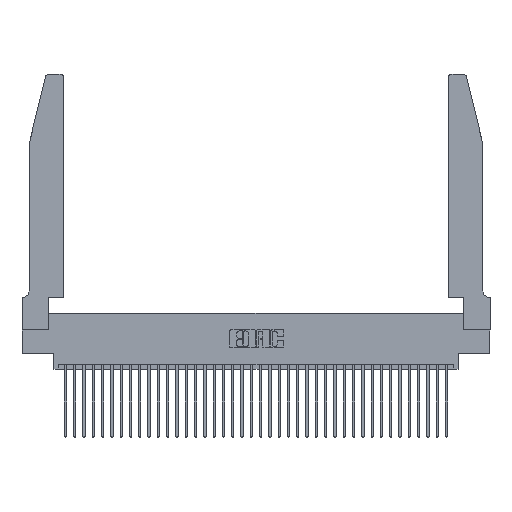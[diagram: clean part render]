
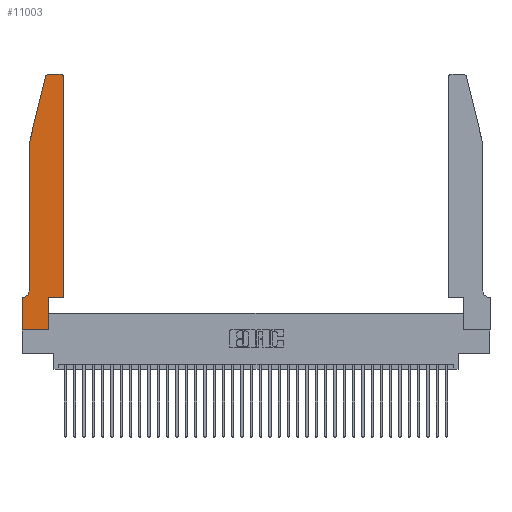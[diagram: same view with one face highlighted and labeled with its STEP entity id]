
A CAD part, top view. The second image highlights one B-rep face of the part: STEP entity #11003.
In plain terms, the highlighted planar face has unit normal (0, 0, 1).
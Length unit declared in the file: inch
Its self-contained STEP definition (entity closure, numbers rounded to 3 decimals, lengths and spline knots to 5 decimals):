
#832 = ORIENTED_EDGE ( 'NONE', *, *, #33440, .T. ) ;
#1424 = EDGE_CURVE ( 'NONE', #3876, #11485, #14101, .T. ) ;
#1878 = VERTEX_POINT ( 'NONE', #6784 ) ;
#2233 = CARTESIAN_POINT ( 'NONE',  ( 0.284, 2.72, 0.37 ) ) ;
#2741 = ORIENTED_EDGE ( 'NONE', *, *, #3928, .T. ) ;
#2839 = AXIS2_PLACEMENT_3D ( 'NONE', #22052, #4454, #24951 ) ;
#3069 = EDGE_CURVE ( 'NONE', #10804, #29101, #21319, .T. ) ;
#3158 = ORIENTED_EDGE ( 'NONE', *, *, #24861, .T. ) ;
#3251 = AXIS2_PLACEMENT_3D ( 'NONE', #17325, #37591, #20279 ) ;
#3876 = VERTEX_POINT ( 'NONE', #34049 ) ;
#3928 = EDGE_CURVE ( 'NONE', #26043, #23030, #18010, .T. ) ;
#4100 = DIRECTION ( 'NONE',  ( 0., 0., 1. ) ) ;
#4180 = CARTESIAN_POINT ( 'NONE',  ( 0.0755, 0.35, 0.37 ) ) ;
#4454 = DIRECTION ( 'NONE',  ( 0., 0., 1. ) ) ;
#5095 = LINE ( 'NONE', #15193, #26618 ) ;
#5207 = DIRECTION ( 'NONE',  ( 1., 0., 0. ) ) ;
#5394 = FACE_OUTER_BOUND ( 'NONE', #14631, .T. ) ;
#5674 = LINE ( 'NONE', #16334, #27212 ) ;
#6263 = VECTOR ( 'NONE', #13726, 39.37008 ) ;
#6784 = CARTESIAN_POINT ( 'NONE',  ( 0.0055, 0.35, 0.37 ) ) ;
#7079 = EDGE_CURVE ( 'NONE', #29101, #33635, #21079, .T. ) ;
#7713 = DIRECTION ( 'NONE',  ( 0., -1., 0. ) ) ;
#7944 = VECTOR ( 'NONE', #7713, 39.37008 ) ;
#9233 = ORIENTED_EDGE ( 'NONE', *, *, #3069, .T. ) ;
#9797 = CARTESIAN_POINT ( 'NONE',  ( 0.25487, 2.72718, 0.37 ) ) ;
#10804 = VERTEX_POINT ( 'NONE', #37589 ) ;
#11003 = ADVANCED_FACE ( 'NONE', ( #5394 ), #12360, .T. ) ;
#11244 = LINE ( 'NONE', #20408, #16251 ) ;
#11485 = VERTEX_POINT ( 'NONE', #24203 ) ;
#11560 = CARTESIAN_POINT ( 'NONE',  ( 0., 0.35, 0.37 ) ) ;
#12360 = PLANE ( 'NONE',  #21242 ) ;
#12640 = DIRECTION ( 'NONE',  ( 1., 0., 0. ) ) ;
#12914 = ORIENTED_EDGE ( 'NONE', *, *, #7079, .T. ) ;
#13045 = CIRCLE ( 'NONE', #3251, 0.07 ) ;
#13524 = VECTOR ( 'NONE', #12640, 39.37008 ) ;
#13726 = DIRECTION ( 'NONE',  ( 0., 1., 0. ) ) ;
#14101 = LINE ( 'NONE', #20466, #6263 ) ;
#14129 = VERTEX_POINT ( 'NONE', #18411 ) ;
#14631 = EDGE_LOOP ( 'NONE', ( #832, #2741, #17920, #18100, #20888, #19071, #25622, #9233, #12914, #26551, #17433, #3158 ) ) ;
#15193 = CARTESIAN_POINT ( 'NONE',  ( 0.4505, 0.35, 0.37 ) ) ;
#15450 = LINE ( 'NONE', #31044, #7944 ) ;
#16251 = VECTOR ( 'NONE', #34852, 39.37008 ) ;
#16334 = CARTESIAN_POINT ( 'NONE',  ( 0.0755, 2., 0.37 ) ) ;
#17325 = CARTESIAN_POINT ( 'NONE',  ( 0.0055, 0.42, 0.37 ) ) ;
#17433 = ORIENTED_EDGE ( 'NONE', *, *, #1424, .T. ) ;
#17920 = ORIENTED_EDGE ( 'NONE', *, *, #19954, .T. ) ;
#17972 = EDGE_CURVE ( 'NONE', #18671, #10804, #11244, .T. ) ;
#18010 = CIRCLE ( 'NONE', #24041, 0.03 ) ;
#18100 = ORIENTED_EDGE ( 'NONE', *, *, #37395, .T. ) ;
#18411 = CARTESIAN_POINT ( 'NONE',  ( 0.0755, 2., 0.37 ) ) ;
#18671 = VERTEX_POINT ( 'NONE', #11560 ) ;
#18738 = VECTOR ( 'NONE', #34705, 39.37008 ) ;
#19071 = ORIENTED_EDGE ( 'NONE', *, *, #31111, .T. ) ;
#19954 = EDGE_CURVE ( 'NONE', #23030, #14129, #5674, .T. ) ;
#20186 = EDGE_CURVE ( 'NONE', #25778, #1878, #13045, .T. ) ;
#20279 = DIRECTION ( 'NONE',  ( -1., 0., 0. ) ) ;
#20408 = CARTESIAN_POINT ( 'NONE',  ( 0., 0., 0.37 ) ) ;
#20466 = CARTESIAN_POINT ( 'NONE',  ( 0.4505, 0.35, 0.37 ) ) ;
#20826 = LINE ( 'NONE', #4180, #34412 ) ;
#20888 = ORIENTED_EDGE ( 'NONE', *, *, #20186, .T. ) ;
#21079 = LINE ( 'NONE', #33098, #36442 ) ;
#21242 = AXIS2_PLACEMENT_3D ( 'NONE', #29795, #4100, #24610 ) ;
#21319 = LINE ( 'NONE', #32979, #13524 ) ;
#21517 = CARTESIAN_POINT ( 'NONE',  ( 0.2865, 0., 0.37 ) ) ;
#21613 = EDGE_CURVE ( 'NONE', #33635, #3876, #5095, .T. ) ;
#22040 = VERTEX_POINT ( 'NONE', #31577 ) ;
#22052 = CARTESIAN_POINT ( 'NONE',  ( 0.4205, 2.72, 0.37 ) ) ;
#22798 = DIRECTION ( 'NONE',  ( 0., 0., 1. ) ) ;
#23030 = VERTEX_POINT ( 'NONE', #9797 ) ;
#24041 = AXIS2_PLACEMENT_3D ( 'NONE', #2233, #22798, #5207 ) ;
#24203 = CARTESIAN_POINT ( 'NONE',  ( 0.4505, 2.72, 0.37 ) ) ;
#24505 = DIRECTION ( 'NONE',  ( 0., 1., 0. ) ) ;
#24610 = DIRECTION ( 'NONE',  ( 1., 0., 0. ) ) ;
#24684 = DIRECTION ( 'NONE',  ( -1., 0., 0. ) ) ;
#24861 = EDGE_CURVE ( 'NONE', #11485, #22040, #33159, .T. ) ;
#24951 = DIRECTION ( 'NONE',  ( 1., 0., 0. ) ) ;
#25622 = ORIENTED_EDGE ( 'NONE', *, *, #17972, .T. ) ;
#25778 = VERTEX_POINT ( 'NONE', #35390 ) ;
#26043 = VERTEX_POINT ( 'NONE', #30576 ) ;
#26111 = CARTESIAN_POINT ( 'NONE',  ( 0.2605, 2.75, 0.37 ) ) ;
#26551 = ORIENTED_EDGE ( 'NONE', *, *, #21613, .T. ) ;
#26618 = VECTOR ( 'NONE', #29723, 39.37008 ) ;
#27212 = VECTOR ( 'NONE', #33741, 39.37008 ) ;
#29101 = VERTEX_POINT ( 'NONE', #21517 ) ;
#29723 = DIRECTION ( 'NONE',  ( 1., 0., 0. ) ) ;
#29795 = CARTESIAN_POINT ( 'NONE',  ( 0., 0.35, 0.37 ) ) ;
#30576 = CARTESIAN_POINT ( 'NONE',  ( 0.284, 2.75, 0.37 ) ) ;
#31044 = CARTESIAN_POINT ( 'NONE',  ( 0.0755, 2., 0.37 ) ) ;
#31111 = EDGE_CURVE ( 'NONE', #1878, #18671, #20826, .T. ) ;
#31577 = CARTESIAN_POINT ( 'NONE',  ( 0.4205, 2.75, 0.37 ) ) ;
#32979 = CARTESIAN_POINT ( 'NONE',  ( 0., 0., 0.37 ) ) ;
#33098 = CARTESIAN_POINT ( 'NONE',  ( 0.2865, 0.35, 0.37 ) ) ;
#33159 = CIRCLE ( 'NONE', #2839, 0.03 ) ;
#33440 = EDGE_CURVE ( 'NONE', #22040, #26043, #35088, .T. ) ;
#33635 = VERTEX_POINT ( 'NONE', #35445 ) ;
#33741 = DIRECTION ( 'NONE',  ( -0.239, -0.971, 0. ) ) ;
#34049 = CARTESIAN_POINT ( 'NONE',  ( 0.4505, 0.35, 0.37 ) ) ;
#34412 = VECTOR ( 'NONE', #24684, 39.37008 ) ;
#34705 = DIRECTION ( 'NONE',  ( -1., 0., 0. ) ) ;
#34852 = DIRECTION ( 'NONE',  ( 0., -1., 0. ) ) ;
#35088 = LINE ( 'NONE', #26111, #18738 ) ;
#35390 = CARTESIAN_POINT ( 'NONE',  ( 0.0755, 0.42, 0.37 ) ) ;
#35445 = CARTESIAN_POINT ( 'NONE',  ( 0.2865, 0.35, 0.37 ) ) ;
#36442 = VECTOR ( 'NONE', #24505, 39.37008 ) ;
#37395 = EDGE_CURVE ( 'NONE', #14129, #25778, #15450, .T. ) ;
#37589 = CARTESIAN_POINT ( 'NONE',  ( 0., 0., 0.37 ) ) ;
#37591 = DIRECTION ( 'NONE',  ( 0., 0., -1. ) ) ;
